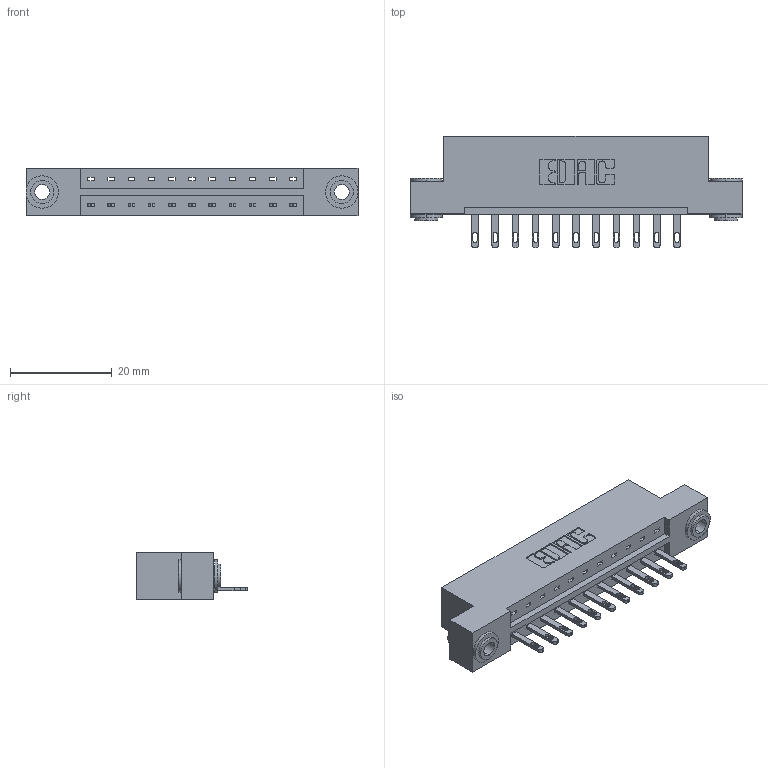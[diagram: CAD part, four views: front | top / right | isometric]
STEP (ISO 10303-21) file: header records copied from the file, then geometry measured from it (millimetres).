
FILE_DESCRIPTION (( 'STEP AP203' ), '1' );
FILE_NAME ('333-011-500-103.STEP', '2018-07-31T23:14:02', ( '' ), ( '' ), 'SwSTEP 2.0', 'SolidWorks 2016', '' );
FILE_SCHEMA (( 'CONFIG_CONTROL_DESIGN' ));
Length unit declared in the file: inch
Products named in the file (4): 333 Part_Flush - .156 Dia - TH; 345-292-001_345-293-100; 345-250-002_345-250-002-102; 333-011-500-103
Assembly tree (14 placements, depth 2):
  333-011-500-103
    333 Part_Flush - .156 Dia - TH
    345-292-001_345-293-100  x11
    345-250-002_345-250-002-102  x2
Bounding box: 65.13 x 21.85 x 9.4 mm (x, y, z)
Volume: 6313.1 mm3; surface area: 6882 mm2
Topology: 14 solids, 14 shells, 746 faces, 2235 edges, 1486 vertices
Faces by surface type: plane 476, cylinder 262, cone 8
Entity records: 11314 total; most frequent: CARTESIAN_POINT 1934, ORIENTED_EDGE 1874, DIRECTION 1729, EDGE_CURVE 937, VECTOR 781, LINE 781, VERTEX_POINT 622, AXIS2_PLACEMENT_3D 474
